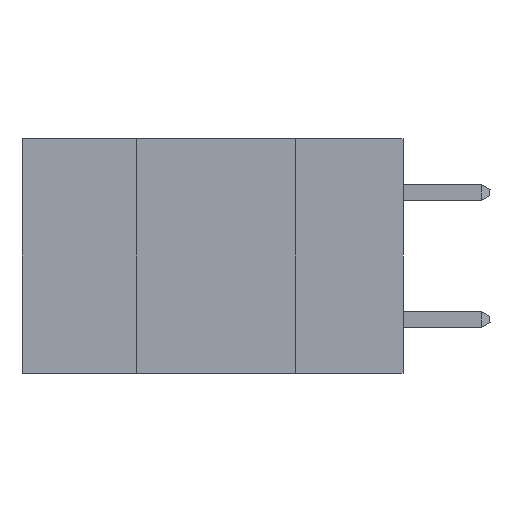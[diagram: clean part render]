
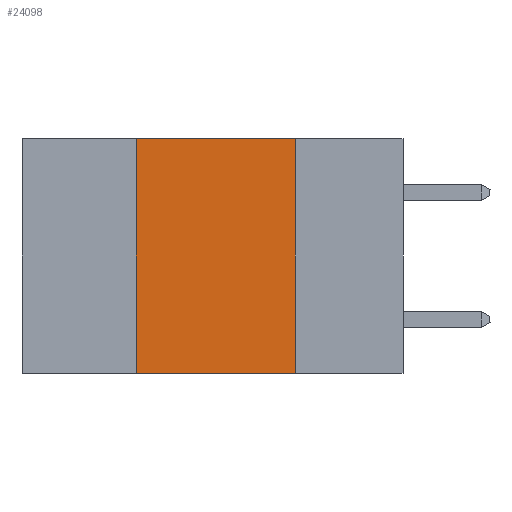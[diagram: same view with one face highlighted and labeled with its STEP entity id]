
A CAD part, left-side view. The second image highlights one B-rep face of the part: STEP entity #24098.
In plain terms, the highlighted planar face has unit normal (-1, 0, 0).
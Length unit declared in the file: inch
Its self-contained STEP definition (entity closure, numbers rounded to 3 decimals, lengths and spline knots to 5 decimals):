
#353 = ORIENTED_EDGE ( 'NONE', *, *, #13046, .F. ) ;
#1177 = DIRECTION ( 'NONE',  ( 1., 0., 0. ) ) ;
#2023 = VECTOR ( 'NONE', #4992, 39.37008 ) ;
#2040 = CARTESIAN_POINT ( 'NONE',  ( 0., 0.17, 0. ) ) ;
#2242 = EDGE_LOOP ( 'NONE', ( #353, #23676, #34470, #13428 ) ) ;
#4992 = DIRECTION ( 'NONE',  ( 0., -1., 0. ) ) ;
#6305 = DIRECTION ( 'NONE',  ( 0., 0., -1. ) ) ;
#6432 = DIRECTION ( 'NONE',  ( 0., 0., -1. ) ) ;
#8599 = LINE ( 'NONE', #24816, #10339 ) ;
#8826 = FACE_OUTER_BOUND ( 'NONE', #2242, .T. ) ;
#9935 = EDGE_CURVE ( 'NONE', #20911, #14742, #17347, .T. ) ;
#10339 = VECTOR ( 'NONE', #26683, 39.37008 ) ;
#12449 = DIRECTION ( 'NONE',  ( 0., -1., 0. ) ) ;
#12967 = AXIS2_PLACEMENT_3D ( 'NONE', #28965, #1177, #6432 ) ;
#13046 = EDGE_CURVE ( 'NONE', #14742, #34234, #27674, .T. ) ;
#13075 = CARTESIAN_POINT ( 'NONE',  ( 0., 0.6, 0. ) ) ;
#13428 = ORIENTED_EDGE ( 'NONE', *, *, #22361, .T. ) ;
#14742 = VERTEX_POINT ( 'NONE', #2040 ) ;
#14947 = EDGE_CURVE ( 'NONE', #19562, #20911, #8599, .T. ) ;
#15091 = PLANE ( 'NONE',  #12967 ) ;
#16697 = CARTESIAN_POINT ( 'NONE',  ( 0., 0.17, -0.37 ) ) ;
#17347 = LINE ( 'NONE', #13075, #2023 ) ;
#19562 = VERTEX_POINT ( 'NONE', #31782 ) ;
#20251 = VECTOR ( 'NONE', #6305, 39.37008 ) ;
#20911 = VERTEX_POINT ( 'NONE', #26935 ) ;
#22361 = EDGE_CURVE ( 'NONE', #19562, #34234, #32978, .T. ) ;
#23676 = ORIENTED_EDGE ( 'NONE', *, *, #9935, .F. ) ;
#24098 = ADVANCED_FACE ( 'NONE', ( #8826 ), #15091, .F. ) ;
#24816 = CARTESIAN_POINT ( 'NONE',  ( 0., 0.42, 0. ) ) ;
#26002 = VECTOR ( 'NONE', #12449, 39.37008 ) ;
#26683 = DIRECTION ( 'NONE',  ( 0., 0., 1. ) ) ;
#26935 = CARTESIAN_POINT ( 'NONE',  ( 0., 0.42, 0. ) ) ;
#27674 = LINE ( 'NONE', #33345, #20251 ) ;
#28965 = CARTESIAN_POINT ( 'NONE',  ( 0., 0.6, 0. ) ) ;
#29001 = CARTESIAN_POINT ( 'NONE',  ( 0., 0.6, -0.37 ) ) ;
#31782 = CARTESIAN_POINT ( 'NONE',  ( 0., 0.42, -0.37 ) ) ;
#32978 = LINE ( 'NONE', #29001, #26002 ) ;
#33345 = CARTESIAN_POINT ( 'NONE',  ( 0., 0.17, 0. ) ) ;
#34234 = VERTEX_POINT ( 'NONE', #16697 ) ;
#34470 = ORIENTED_EDGE ( 'NONE', *, *, #14947, .F. ) ;
